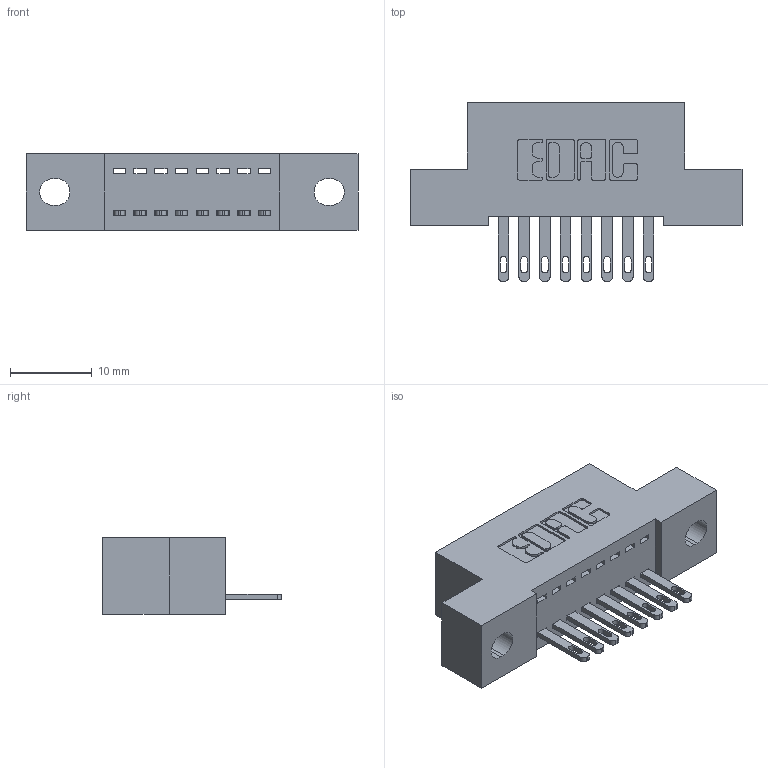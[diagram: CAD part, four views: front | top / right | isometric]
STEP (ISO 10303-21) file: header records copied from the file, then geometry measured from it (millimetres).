
FILE_DESCRIPTION (( 'STEP AP203' ), '1' );
FILE_NAME ('342-008-500-102.STEP', '2019-10-01T13:00:49', ( '' ), ( '' ), 'SwSTEP 2.0', 'SolidWorks 2016', '' );
FILE_SCHEMA (( 'CONFIG_CONTROL_DESIGN' ));
Length unit declared in the file: inch
Products named in the file (3): 342-008-500-102; 342 Part_.128 Slot; 345-292-001_345-293-100
Assembly tree (9 placements, depth 2):
  342-008-500-102
    342 Part_.128 Slot
    345-292-001_345-293-100  x8
Bounding box: 40.64 x 21.85 x 9.4 mm (x, y, z)
Volume: 3390.9 mm3; surface area: 4119.9 mm2
Topology: 9 solids, 9 shells, 546 faces, 1655 edges, 1102 vertices
Faces by surface type: plane 358, cylinder 188
Entity records: 9221 total; most frequent: CARTESIAN_POINT 1602, ORIENTED_EDGE 1546, DIRECTION 1421, EDGE_CURVE 773, VECTOR 641, LINE 641, VERTEX_POINT 514, AXIS2_PLACEMENT_3D 390
